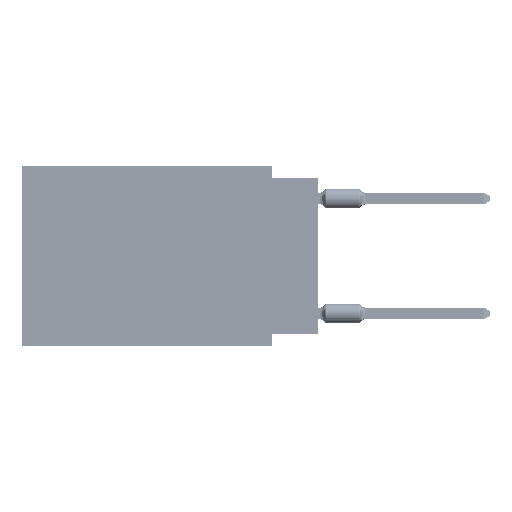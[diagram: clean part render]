
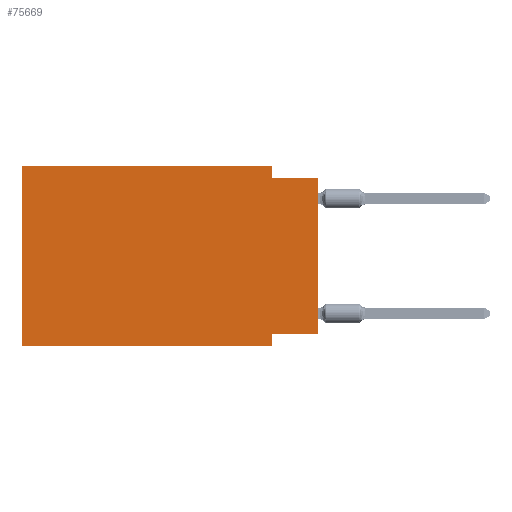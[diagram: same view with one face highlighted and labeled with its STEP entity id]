
A CAD part, left-side view. The second image highlights one B-rep face of the part: STEP entity #75669.
In plain terms, the highlighted planar face has unit normal (-1, 0, 0).
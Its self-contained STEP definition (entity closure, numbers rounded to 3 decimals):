
#805 = CARTESIAN_POINT ( 'NONE',  ( 0., 16.383, 0. ) ) ;
#828 = CARTESIAN_POINT ( 'NONE',  ( 0., 2.54, -9.271 ) ) ;
#1263 = CARTESIAN_POINT ( 'NONE',  ( 0., 16.383, -9.906 ) ) ;
#1732 = CARTESIAN_POINT ( 'NONE',  ( 0., 16.383, 0. ) ) ;
#1902 = ORIENTED_EDGE ( 'NONE', *, *, #71391, .F. ) ;
#3575 = DIRECTION ( 'NONE',  ( 0., 0., 1. ) ) ;
#3740 = CARTESIAN_POINT ( 'NONE',  ( 0., 0., 0. ) ) ;
#3802 = LINE ( 'NONE', #72414, #54815 ) ;
#4095 = VECTOR ( 'NONE', #78342, 1000. ) ;
#4992 = VECTOR ( 'NONE', #8439, 1000. ) ;
#6461 = ORIENTED_EDGE ( 'NONE', *, *, #82601, .T. ) ;
#7426 = CARTESIAN_POINT ( 'NONE',  ( 0., 2.54, -0.635 ) ) ;
#7530 = PLANE ( 'NONE',  #53274 ) ;
#8026 = EDGE_CURVE ( 'NONE', #26433, #43545, #3802, .T. ) ;
#8439 = DIRECTION ( 'NONE',  ( 0., -1., 0. ) ) ;
#10664 = VECTOR ( 'NONE', #60135, 1000. ) ;
#15123 = FACE_OUTER_BOUND ( 'NONE', #23148, .T. ) ;
#15919 = DIRECTION ( 'NONE',  ( 0., 0., -1. ) ) ;
#21784 = VECTOR ( 'NONE', #15919, 1000. ) ;
#23148 = EDGE_LOOP ( 'NONE', ( #6461, #47625, #41919, #64348, #72367, #86478, #34257, #1902 ) ) ;
#24097 = VERTEX_POINT ( 'NONE', #51346 ) ;
#26433 = VERTEX_POINT ( 'NONE', #828 ) ;
#27591 = LINE ( 'NONE', #43300, #21784 ) ;
#27865 = VERTEX_POINT ( 'NONE', #7426 ) ;
#30389 = DIRECTION ( 'NONE',  ( 0., 0., -1. ) ) ;
#32289 = EDGE_CURVE ( 'NONE', #77405, #27865, #27591, .T. ) ;
#32781 = LINE ( 'NONE', #73625, #10664 ) ;
#34257 = ORIENTED_EDGE ( 'NONE', *, *, #8026, .F. ) ;
#36591 = VERTEX_POINT ( 'NONE', #1263 ) ;
#37518 = LINE ( 'NONE', #43356, #4095 ) ;
#38692 = LINE ( 'NONE', #54304, #44579 ) ;
#39587 = VERTEX_POINT ( 'NONE', #79646 ) ;
#40555 = VERTEX_POINT ( 'NONE', #66226 ) ;
#41919 = ORIENTED_EDGE ( 'NONE', *, *, #32289, .F. ) ;
#43236 = EDGE_CURVE ( 'NONE', #39587, #77405, #76623, .T. ) ;
#43300 = CARTESIAN_POINT ( 'NONE',  ( 0., 2.54, 0. ) ) ;
#43356 = CARTESIAN_POINT ( 'NONE',  ( 0., 0., -9.271 ) ) ;
#43545 = VERTEX_POINT ( 'NONE', #68452 ) ;
#44579 = VECTOR ( 'NONE', #46706, 1000. ) ;
#44821 = LINE ( 'NONE', #52415, #86463 ) ;
#46706 = DIRECTION ( 'NONE',  ( 0., -1., 0. ) ) ;
#47625 = ORIENTED_EDGE ( 'NONE', *, *, #66335, .F. ) ;
#50953 = EDGE_CURVE ( 'NONE', #36591, #43545, #38692, .T. ) ;
#51276 = DIRECTION ( 'NONE',  ( 0., 0., 1. ) ) ;
#51346 = CARTESIAN_POINT ( 'NONE',  ( 0., 0., -0.635 ) ) ;
#51375 = CARTESIAN_POINT ( 'NONE',  ( 0., 2.54, 0. ) ) ;
#52415 = CARTESIAN_POINT ( 'NONE',  ( 0., 16.383, 0. ) ) ;
#53274 = AXIS2_PLACEMENT_3D ( 'NONE', #805, #62687, #30389 ) ;
#54304 = CARTESIAN_POINT ( 'NONE',  ( 0., 16.383, -9.906 ) ) ;
#54815 = VECTOR ( 'NONE', #81686, 1000. ) ;
#60135 = DIRECTION ( 'NONE',  ( 0., -1., 0. ) ) ;
#62687 = DIRECTION ( 'NONE',  ( 1., 0., 0. ) ) ;
#64348 = ORIENTED_EDGE ( 'NONE', *, *, #43236, .F. ) ;
#64976 = EDGE_CURVE ( 'NONE', #36591, #39587, #44821, .T. ) ;
#66226 = CARTESIAN_POINT ( 'NONE',  ( 0., 0., -9.271 ) ) ;
#66335 = EDGE_CURVE ( 'NONE', #27865, #24097, #32781, .T. ) ;
#68452 = CARTESIAN_POINT ( 'NONE',  ( 0., 2.54, -9.906 ) ) ;
#71391 = EDGE_CURVE ( 'NONE', #40555, #26433, #37518, .T. ) ;
#72355 = LINE ( 'NONE', #3740, #88082 ) ;
#72367 = ORIENTED_EDGE ( 'NONE', *, *, #64976, .F. ) ;
#72414 = CARTESIAN_POINT ( 'NONE',  ( 0., 2.54, -9.906 ) ) ;
#73625 = CARTESIAN_POINT ( 'NONE',  ( 0., 0., -0.635 ) ) ;
#75669 = ADVANCED_FACE ( 'NONE', ( #15123 ), #7530, .F. ) ;
#76623 = LINE ( 'NONE', #1732, #4992 ) ;
#77405 = VERTEX_POINT ( 'NONE', #51375 ) ;
#78342 = DIRECTION ( 'NONE',  ( 0., 1., 0. ) ) ;
#79646 = CARTESIAN_POINT ( 'NONE',  ( 0., 16.383, 0. ) ) ;
#81686 = DIRECTION ( 'NONE',  ( 0., 0., -1. ) ) ;
#82601 = EDGE_CURVE ( 'NONE', #40555, #24097, #72355, .T. ) ;
#86463 = VECTOR ( 'NONE', #3575, 1000. ) ;
#86478 = ORIENTED_EDGE ( 'NONE', *, *, #50953, .T. ) ;
#88082 = VECTOR ( 'NONE', #51276, 1000. ) ;
